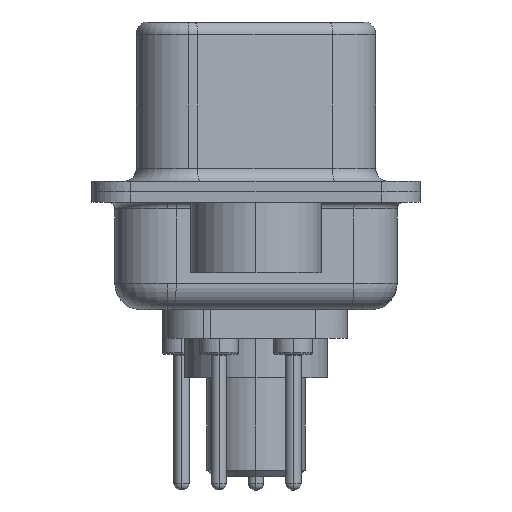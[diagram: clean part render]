
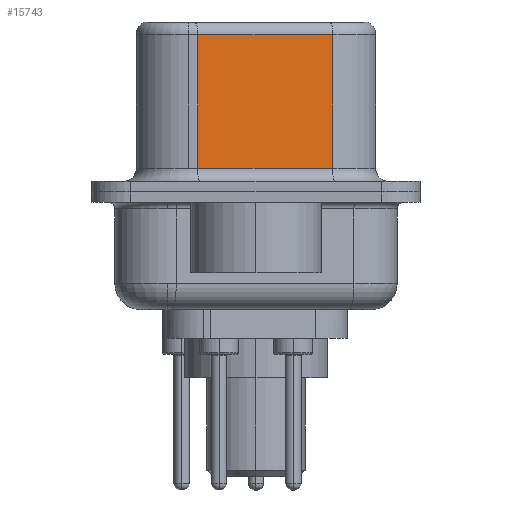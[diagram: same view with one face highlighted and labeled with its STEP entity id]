
A CAD part, left-side view. The second image highlights one B-rep face of the part: STEP entity #15743.
In plain terms, the highlighted planar face has unit normal (-0.985, -0.174, 0).
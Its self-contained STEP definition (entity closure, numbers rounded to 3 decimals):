
#1188 = CARTESIAN_POINT ( 'NONE',  ( 4.585, -2.927, 0.9 ) ) ;
#1275 = EDGE_CURVE ( 'NONE', #14692, #9295, #16764, .T. ) ;
#1290 = CARTESIAN_POINT ( 'NONE',  ( 4.585, -2.927, 0.9 ) ) ;
#1438 = CARTESIAN_POINT ( 'NONE',  ( 4.585, -2.927, 6.52 ) ) ;
#2397 = CARTESIAN_POINT ( 'NONE',  ( 3.675, 2.233, 6.52 ) ) ;
#2500 = DIRECTION ( 'NONE',  ( 0.174, -0.985, 0. ) ) ;
#2973 = LINE ( 'NONE', #3578, #3273 ) ;
#3053 = DIRECTION ( 'NONE',  ( -0.174, 0.985, 0. ) ) ;
#3273 = VECTOR ( 'NONE', #17918, 1000. ) ;
#3578 = CARTESIAN_POINT ( 'NONE',  ( 4.585, -2.927, 6.52 ) ) ;
#3759 = EDGE_CURVE ( 'NONE', #14525, #14692, #5935, .T. ) ;
#4741 = AXIS2_PLACEMENT_3D ( 'NONE', #1438, #6795, #3053 ) ;
#5935 = LINE ( 'NONE', #21071, #11344 ) ;
#6735 = DIRECTION ( 'NONE',  ( -0.174, 0.985, 0. ) ) ;
#6795 = DIRECTION ( 'NONE',  ( 0.985, 0.174, 0. ) ) ;
#7474 = VECTOR ( 'NONE', #14922, 1000. ) ;
#8530 = PLANE ( 'NONE',  #4741 ) ;
#8733 = EDGE_CURVE ( 'NONE', #14525, #17447, #2973, .T. ) ;
#9181 = ORIENTED_EDGE ( 'NONE', *, *, #18669, .T. ) ;
#9295 = VERTEX_POINT ( 'NONE', #21069 ) ;
#9950 = FACE_OUTER_BOUND ( 'NONE', #18929, .T. ) ;
#11344 = VECTOR ( 'NONE', #6735, 1000. ) ;
#14525 = VERTEX_POINT ( 'NONE', #22742 ) ;
#14692 = VERTEX_POINT ( 'NONE', #17908 ) ;
#14922 = DIRECTION ( 'NONE',  ( 0., 0., -1. ) ) ;
#15743 = ADVANCED_FACE ( 'NONE', ( #9950 ), #8530, .F. ) ;
#16764 = LINE ( 'NONE', #2397, #7474 ) ;
#16769 = ORIENTED_EDGE ( 'NONE', *, *, #8733, .F. ) ;
#16788 = ORIENTED_EDGE ( 'NONE', *, *, #1275, .T. ) ;
#17447 = VERTEX_POINT ( 'NONE', #1290 ) ;
#17908 = CARTESIAN_POINT ( 'NONE',  ( 3.675, 2.233, 6.02 ) ) ;
#17918 = DIRECTION ( 'NONE',  ( 0., 0., -1. ) ) ;
#18669 = EDGE_CURVE ( 'NONE', #9295, #17447, #21684, .T. ) ;
#18929 = EDGE_LOOP ( 'NONE', ( #16769, #19914, #16788, #9181 ) ) ;
#19452 = VECTOR ( 'NONE', #2500, 1000. ) ;
#19914 = ORIENTED_EDGE ( 'NONE', *, *, #3759, .T. ) ;
#21069 = CARTESIAN_POINT ( 'NONE',  ( 3.675, 2.233, 0.9 ) ) ;
#21071 = CARTESIAN_POINT ( 'NONE',  ( 4.585, -2.927, 6.02 ) ) ;
#21684 = LINE ( 'NONE', #1188, #19452 ) ;
#22742 = CARTESIAN_POINT ( 'NONE',  ( 4.585, -2.927, 6.02 ) ) ;
